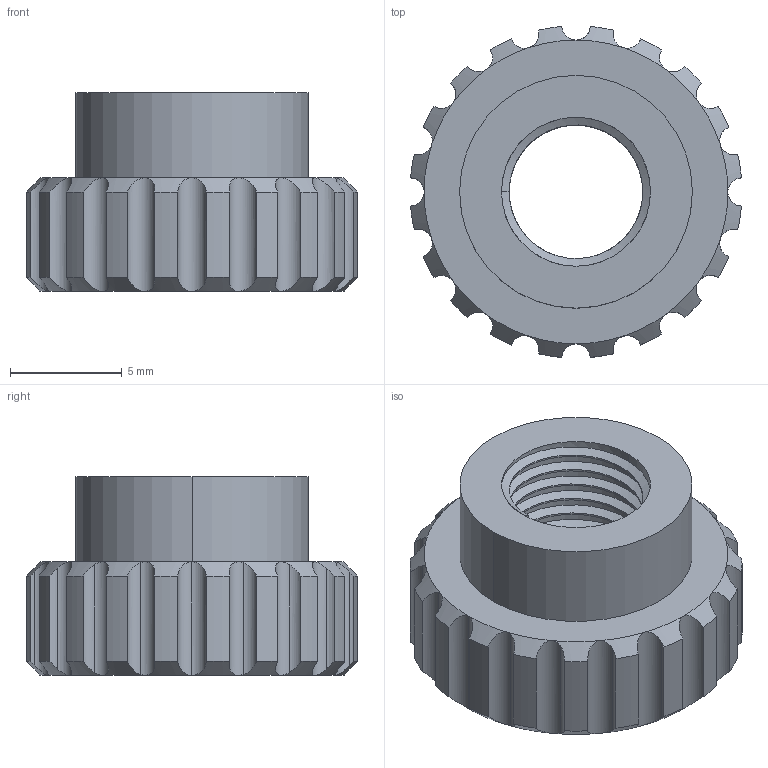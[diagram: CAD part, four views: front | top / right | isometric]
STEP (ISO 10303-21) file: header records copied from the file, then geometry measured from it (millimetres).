
FILE_DESCRIPTION (( 'STEP AP203' ), '1' );
FILE_NAME ('AF-WF-GS-PRT-010-STEP.STEP', '2020-07-21T19:14:32', ( '' ), ( '' ), 'SwSTEP 2.0', 'SolidWorks 2018', '' );
FILE_SCHEMA (( 'CONFIG_CONTROL_DESIGN' ));
Length unit declared in the file: inch
Products named in the file (1): AF-WF-GS-PRT-010-STEP
Bounding box: 14.8 x 14.8 x 8.89 mm (x, y, z)
Volume: 842.8 mm3; surface area: 912 mm2
Topology: 1 solids, 1 shells, 121 faces, 309 edges, 191 vertices
Faces by surface type: cylinder 73, cone 40, plane 5, bspline 3
Entity records: 5708 total; most frequent: CARTESIAN_POINT 2987, ORIENTED_EDGE 618, DIRECTION 489, EDGE_CURVE 309, AXIS2_PLACEMENT_3D 207, VERTEX_POINT 191, EDGE_LOOP 124, FACE_OUTER_BOUND 121
